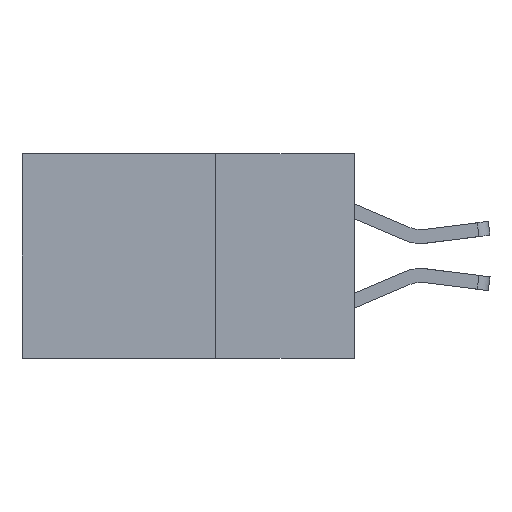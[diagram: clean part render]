
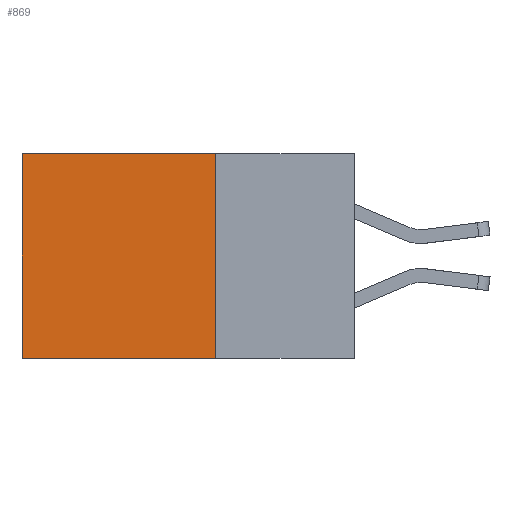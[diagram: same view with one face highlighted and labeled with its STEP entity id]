
A CAD part, left-side view. The second image highlights one B-rep face of the part: STEP entity #869.
In plain terms, the highlighted planar face has unit normal (-1, 0, 0).
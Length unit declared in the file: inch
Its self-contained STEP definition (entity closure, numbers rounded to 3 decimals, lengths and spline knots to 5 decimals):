
#166 = VERTEX_POINT ( 'NONE', #11160 ) ;
#301 = VECTOR ( 'NONE', #7458, 39.37008 ) ;
#321 = ORIENTED_EDGE ( 'NONE', *, *, #1276, .T. ) ;
#510 = EDGE_LOOP ( 'NONE', ( #10918, #7433, #7745, #321 ) ) ;
#869 = ADVANCED_FACE ( 'NONE', ( #3415 ), #2988, .F. ) ;
#1276 = EDGE_CURVE ( 'NONE', #7904, #166, #6343, .T. ) ;
#1310 = CARTESIAN_POINT ( 'NONE',  ( 0.298, 0.25, -0.37 ) ) ;
#2010 = DIRECTION ( 'NONE',  ( 1., 0., 0. ) ) ;
#2027 = AXIS2_PLACEMENT_3D ( 'NONE', #5580, #2010, #3793 ) ;
#2357 = CARTESIAN_POINT ( 'NONE',  ( 0.298, 0.25, 0. ) ) ;
#2389 = DIRECTION ( 'NONE',  ( 0., 0., -1. ) ) ;
#2811 = CARTESIAN_POINT ( 'NONE',  ( 0.298, 0.25, 0. ) ) ;
#2988 = PLANE ( 'NONE',  #2027 ) ;
#3179 = VERTEX_POINT ( 'NONE', #10908 ) ;
#3415 = FACE_OUTER_BOUND ( 'NONE', #510, .T. ) ;
#3792 = LINE ( 'NONE', #4584, #11052 ) ;
#3793 = DIRECTION ( 'NONE',  ( 0., 0., -1. ) ) ;
#3972 = VERTEX_POINT ( 'NONE', #5707 ) ;
#4162 = EDGE_CURVE ( 'NONE', #3179, #3972, #7360, .T. ) ;
#4496 = DIRECTION ( 'NONE',  ( 0., 0., -1. ) ) ;
#4584 = CARTESIAN_POINT ( 'NONE',  ( 0.298, 0.6, 0. ) ) ;
#4832 = VECTOR ( 'NONE', #8025, 39.37008 ) ;
#5207 = VECTOR ( 'NONE', #2389, 39.37008 ) ;
#5580 = CARTESIAN_POINT ( 'NONE',  ( 0.298, 0.25, 0. ) ) ;
#5707 = CARTESIAN_POINT ( 'NONE',  ( 0.298, 0.6, -0.37 ) ) ;
#6278 = EDGE_CURVE ( 'NONE', #166, #3972, #3792, .T. ) ;
#6343 = LINE ( 'NONE', #2811, #4832 ) ;
#7360 = LINE ( 'NONE', #1310, #301 ) ;
#7433 = ORIENTED_EDGE ( 'NONE', *, *, #4162, .F. ) ;
#7458 = DIRECTION ( 'NONE',  ( 0., 1., 0. ) ) ;
#7745 = ORIENTED_EDGE ( 'NONE', *, *, #7802, .F. ) ;
#7802 = EDGE_CURVE ( 'NONE', #7904, #3179, #9379, .T. ) ;
#7904 = VERTEX_POINT ( 'NONE', #11407 ) ;
#8025 = DIRECTION ( 'NONE',  ( 0., 1., 0. ) ) ;
#9379 = LINE ( 'NONE', #2357, #5207 ) ;
#10908 = CARTESIAN_POINT ( 'NONE',  ( 0.298, 0.25, -0.37 ) ) ;
#10918 = ORIENTED_EDGE ( 'NONE', *, *, #6278, .T. ) ;
#11052 = VECTOR ( 'NONE', #4496, 39.37008 ) ;
#11160 = CARTESIAN_POINT ( 'NONE',  ( 0.298, 0.6, 0. ) ) ;
#11407 = CARTESIAN_POINT ( 'NONE',  ( 0.298, 0.25, 0. ) ) ;
